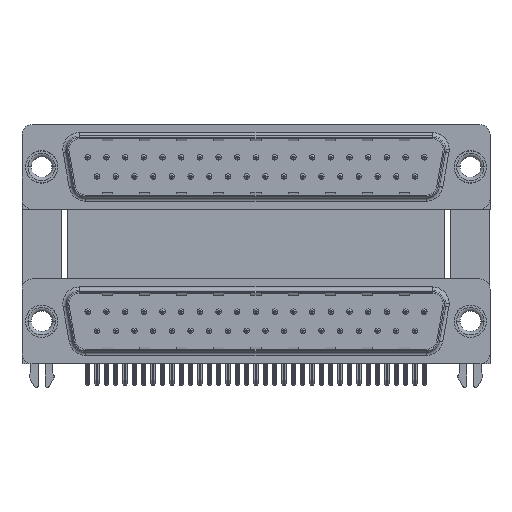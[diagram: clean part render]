
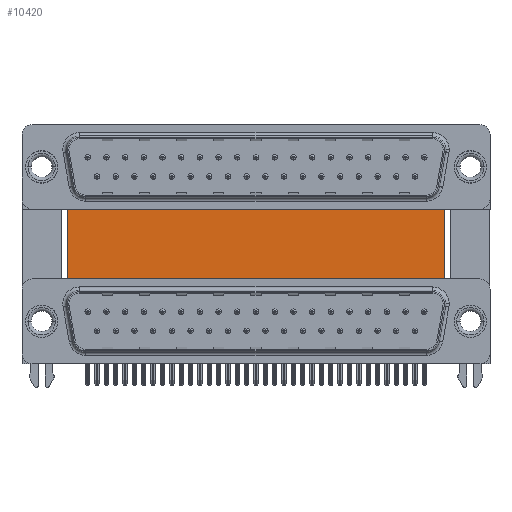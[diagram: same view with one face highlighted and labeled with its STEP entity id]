
A CAD part, top view. The second image highlights one B-rep face of the part: STEP entity #10420.
In plain terms, the highlighted planar face has unit normal (0, 0, 1).
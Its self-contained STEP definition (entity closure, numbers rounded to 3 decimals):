
#233 = ORIENTED_EDGE ( 'NONE', *, *, #50042, .T. ) ;
#493 = PLANE ( 'NONE',  #35925 ) ;
#591 = LINE ( 'NONE', #27466, #21128 ) ;
#747 = DIRECTION ( 'NONE',  ( 0., 0., -1. ) ) ;
#2026 = VECTOR ( 'NONE', #41352, 1000. ) ;
#3751 = VECTOR ( 'NONE', #15610, 1000. ) ;
#5729 = EDGE_LOOP ( 'NONE', ( #48158, #49073, #48989, #233 ) ) ;
#7823 = CARTESIAN_POINT ( 'NONE',  ( 59.71, 16.585, -12. ) ) ;
#8815 = VERTEX_POINT ( 'NONE', #21434 ) ;
#9880 = CARTESIAN_POINT ( 'NONE',  ( 3.79, -3.735, -12. ) ) ;
#9947 = CARTESIAN_POINT ( 'NONE',  ( 3.79, 16.585, -12. ) ) ;
#10420 = ADVANCED_FACE ( 'NONE', ( #47970 ), #493, .F. ) ;
#15610 = DIRECTION ( 'NONE',  ( 0., -1., 0. ) ) ;
#16300 = VERTEX_POINT ( 'NONE', #30309 ) ;
#16357 = EDGE_CURVE ( 'NONE', #8815, #47548, #591, .T. ) ;
#17953 = EDGE_CURVE ( 'NONE', #16300, #47942, #29491, .T. ) ;
#21128 = VECTOR ( 'NONE', #47070, 1000. ) ;
#21434 = CARTESIAN_POINT ( 'NONE',  ( 3.79, 16.585, -12. ) ) ;
#25688 = DIRECTION ( 'NONE',  ( 0., -1., 0. ) ) ;
#26860 = EDGE_CURVE ( 'NONE', #47548, #47942, #28208, .T. ) ;
#27466 = CARTESIAN_POINT ( 'NONE',  ( 3.79, 16.585, -12. ) ) ;
#28208 = LINE ( 'NONE', #39816, #3751 ) ;
#29491 = LINE ( 'NONE', #9880, #2026 ) ;
#30309 = CARTESIAN_POINT ( 'NONE',  ( 3.79, -3.735, -12. ) ) ;
#31452 = CARTESIAN_POINT ( 'NONE',  ( 59.71, -3.735, -12. ) ) ;
#35925 = AXIS2_PLACEMENT_3D ( 'NONE', #36593, #747, #47731 ) ;
#36593 = CARTESIAN_POINT ( 'NONE',  ( 3.79, 16.585, -12. ) ) ;
#39816 = CARTESIAN_POINT ( 'NONE',  ( 59.71, 16.585, -12. ) ) ;
#41352 = DIRECTION ( 'NONE',  ( 1., 0., 0. ) ) ;
#41419 = LINE ( 'NONE', #9947, #49806 ) ;
#47070 = DIRECTION ( 'NONE',  ( 1., 0., 0. ) ) ;
#47548 = VERTEX_POINT ( 'NONE', #7823 ) ;
#47731 = DIRECTION ( 'NONE',  ( -1., 0., 0. ) ) ;
#47942 = VERTEX_POINT ( 'NONE', #31452 ) ;
#47970 = FACE_OUTER_BOUND ( 'NONE', #5729, .T. ) ;
#48158 = ORIENTED_EDGE ( 'NONE', *, *, #17953, .T. ) ;
#48989 = ORIENTED_EDGE ( 'NONE', *, *, #16357, .F. ) ;
#49073 = ORIENTED_EDGE ( 'NONE', *, *, #26860, .F. ) ;
#49806 = VECTOR ( 'NONE', #25688, 1000. ) ;
#50042 = EDGE_CURVE ( 'NONE', #8815, #16300, #41419, .T. ) ;
